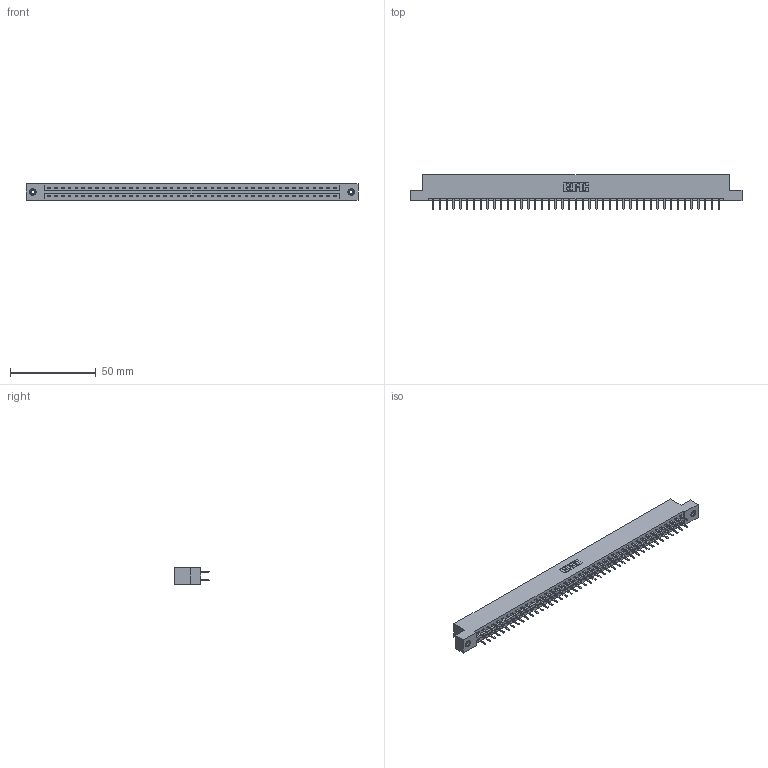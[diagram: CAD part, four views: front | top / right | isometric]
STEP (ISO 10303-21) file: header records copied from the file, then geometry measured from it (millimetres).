
FILE_DESCRIPTION (( 'STEP AP203' ), '1' );
FILE_NAME ('387-086-520-208.STEP', '2019-10-23T02:44:14', ( '' ), ( '' ), 'SwSTEP 2.0', 'SolidWorks 2016', '' );
FILE_SCHEMA (( 'CONFIG_CONTROL_DESIGN' ));
Length unit declared in the file: inch
Products named in the file (4): 337 Part_Flush Mounting Lugs - 0.156 Dia-TI; 345-292-001_345-293-120; 387-086-520-208; 345-250-001_345-250-003-102
Assembly tree (89 placements, depth 2):
  387-086-520-208
    337 Part_Flush Mounting Lugs - 0.156 Dia-TI
    345-292-001_345-293-120  x86
    345-250-001_345-250-003-102  x2
Bounding box: 193.4 x 20.02 x 9.4 mm (x, y, z)
Volume: 20350.5 mm3; surface area: 22932.1 mm2
Topology: 89 solids, 89 shells, 5162 faces, 14981 edges, 9750 vertices
Faces by surface type: plane 3542, cylinder 1604, cone 12, torus 4
Entity records: 34510 total; most frequent: CARTESIAN_POINT 5805, ORIENTED_EDGE 5722, DIRECTION 4955, EDGE_CURVE 2861, VECTOR 2709, LINE 2709, VERTEX_POINT 1900, AXIS2_PLACEMENT_3D 1123
